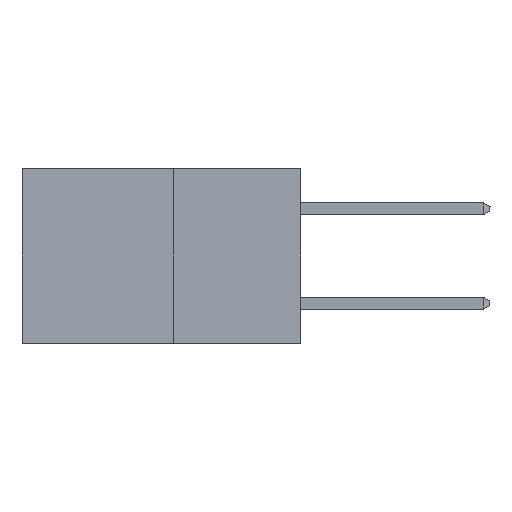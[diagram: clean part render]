
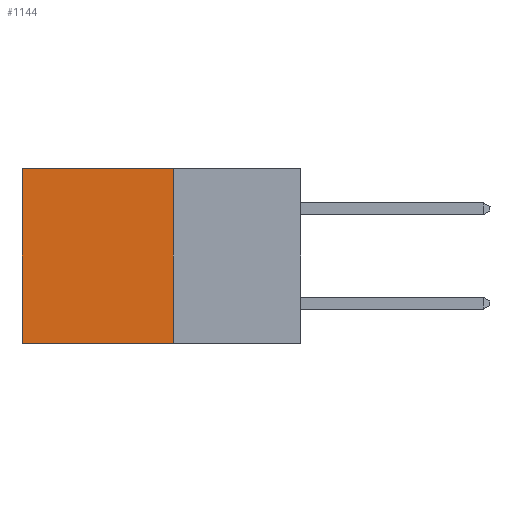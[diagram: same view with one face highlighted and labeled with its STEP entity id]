
A CAD part, left-side view. The second image highlights one B-rep face of the part: STEP entity #1144.
In plain terms, the highlighted planar face has unit normal (-1, 0, 0).
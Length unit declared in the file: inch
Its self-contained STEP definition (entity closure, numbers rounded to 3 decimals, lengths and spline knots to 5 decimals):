
#190 = VERTEX_POINT ( 'NONE', #9649 ) ;
#1132 = VECTOR ( 'NONE', #9918, 39.37008 ) ;
#1144 = ADVANCED_FACE ( 'NONE', ( #5697 ), #2993, .F. ) ;
#1330 = DIRECTION ( 'NONE',  ( 1., 0., 0. ) ) ;
#1406 = EDGE_CURVE ( 'NONE', #190, #9037, #9431, .T. ) ;
#1426 = CARTESIAN_POINT ( 'NONE',  ( 0.277, 0.27, -0.37 ) ) ;
#1443 = CARTESIAN_POINT ( 'NONE',  ( 0.277, 0.59, -0.37 ) ) ;
#1740 = EDGE_CURVE ( 'NONE', #5726, #190, #8840, .T. ) ;
#1766 = VECTOR ( 'NONE', #2507, 39.37008 ) ;
#1794 = DIRECTION ( 'NONE',  ( 0., 0., -1. ) ) ;
#2505 = CARTESIAN_POINT ( 'NONE',  ( 0.277, 0.27, 0. ) ) ;
#2507 = DIRECTION ( 'NONE',  ( 0., 1., 0. ) ) ;
#2631 = DIRECTION ( 'NONE',  ( 0., 0., -1. ) ) ;
#2993 = PLANE ( 'NONE',  #5853 ) ;
#3164 = ORIENTED_EDGE ( 'NONE', *, *, #3952, .T. ) ;
#3341 = LINE ( 'NONE', #7572, #9265 ) ;
#3952 = EDGE_CURVE ( 'NONE', #9455, #9037, #3341, .T. ) ;
#4051 = ORIENTED_EDGE ( 'NONE', *, *, #1406, .F. ) ;
#4539 = ORIENTED_EDGE ( 'NONE', *, *, #1740, .F. ) ;
#4717 = VECTOR ( 'NONE', #1794, 39.37008 ) ;
#5187 = ORIENTED_EDGE ( 'NONE', *, *, #8466, .T. ) ;
#5326 = CARTESIAN_POINT ( 'NONE',  ( 0.277, 0.27, 0. ) ) ;
#5641 = CARTESIAN_POINT ( 'NONE',  ( 0.277, 0.27, -0.37 ) ) ;
#5697 = FACE_OUTER_BOUND ( 'NONE', #9483, .T. ) ;
#5726 = VERTEX_POINT ( 'NONE', #5326 ) ;
#5853 = AXIS2_PLACEMENT_3D ( 'NONE', #1426, #1330, #9379 ) ;
#5927 = LINE ( 'NONE', #2505, #1766 ) ;
#7150 = CARTESIAN_POINT ( 'NONE',  ( 0.277, 0.27, -0.37 ) ) ;
#7572 = CARTESIAN_POINT ( 'NONE',  ( 0.277, 0.59, -0.37 ) ) ;
#8182 = CARTESIAN_POINT ( 'NONE',  ( 0.277, 0.59, 0. ) ) ;
#8466 = EDGE_CURVE ( 'NONE', #5726, #9455, #5927, .T. ) ;
#8840 = LINE ( 'NONE', #5641, #4717 ) ;
#9037 = VERTEX_POINT ( 'NONE', #1443 ) ;
#9265 = VECTOR ( 'NONE', #2631, 39.37008 ) ;
#9379 = DIRECTION ( 'NONE',  ( 0., 0., -1. ) ) ;
#9431 = LINE ( 'NONE', #7150, #1132 ) ;
#9455 = VERTEX_POINT ( 'NONE', #8182 ) ;
#9483 = EDGE_LOOP ( 'NONE', ( #3164, #4051, #4539, #5187 ) ) ;
#9649 = CARTESIAN_POINT ( 'NONE',  ( 0.277, 0.27, -0.37 ) ) ;
#9918 = DIRECTION ( 'NONE',  ( 0., 1., 0. ) ) ;
